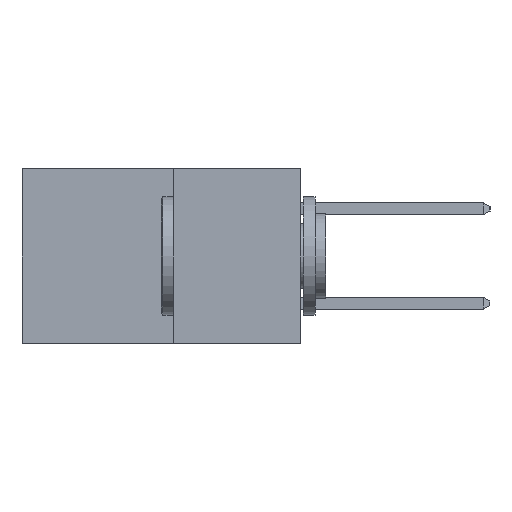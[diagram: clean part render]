
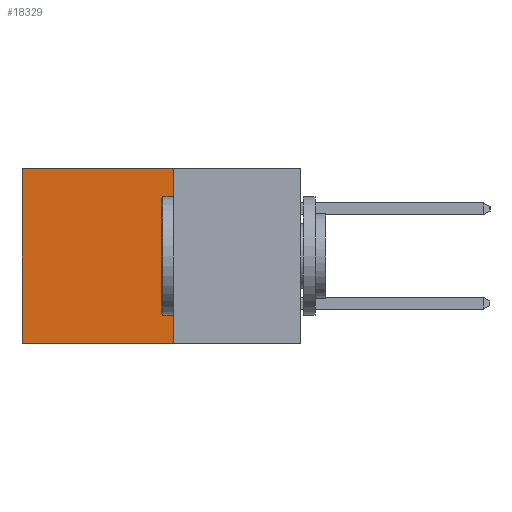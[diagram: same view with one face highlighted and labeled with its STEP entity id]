
A CAD part, left-side view. The second image highlights one B-rep face of the part: STEP entity #18329.
In plain terms, the highlighted planar face has unit normal (-1, 0, 0).
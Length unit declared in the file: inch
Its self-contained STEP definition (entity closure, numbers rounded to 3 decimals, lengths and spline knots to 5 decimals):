
#152 = EDGE_CURVE ( 'NONE', #6228, #7669, #28660, .T. ) ;
#1221 = CARTESIAN_POINT ( 'NONE',  ( 0.277, 0.27, -0.37 ) ) ;
#1982 = PLANE ( 'NONE',  #23885 ) ;
#2943 = DIRECTION ( 'NONE',  ( 0., 1., 0. ) ) ;
#3325 = DIRECTION ( 'NONE',  ( 0., 0., -1. ) ) ;
#4357 = DIRECTION ( 'NONE',  ( 0., 0., -1. ) ) ;
#4383 = ORIENTED_EDGE ( 'NONE', *, *, #19070, .F. ) ;
#5426 = CARTESIAN_POINT ( 'NONE',  ( 0.277, 0.59, -0.37 ) ) ;
#6228 = VERTEX_POINT ( 'NONE', #18841 ) ;
#7325 = FACE_OUTER_BOUND ( 'NONE', #9480, .T. ) ;
#7669 = VERTEX_POINT ( 'NONE', #28360 ) ;
#9480 = EDGE_LOOP ( 'NONE', ( #26126, #4383, #11478, #27191 ) ) ;
#9763 = EDGE_CURVE ( 'NONE', #6228, #13042, #27057, .T. ) ;
#10305 = VERTEX_POINT ( 'NONE', #5426 ) ;
#11478 = ORIENTED_EDGE ( 'NONE', *, *, #9763, .F. ) ;
#13042 = VERTEX_POINT ( 'NONE', #14444 ) ;
#14444 = CARTESIAN_POINT ( 'NONE',  ( 0.277, 0.27, -0.37 ) ) ;
#14736 = CARTESIAN_POINT ( 'NONE',  ( 0.277, 0.27, 0. ) ) ;
#15984 = EDGE_CURVE ( 'NONE', #7669, #10305, #28561, .T. ) ;
#17325 = CARTESIAN_POINT ( 'NONE',  ( 0.277, 0.27, -0.37 ) ) ;
#17965 = DIRECTION ( 'NONE',  ( 0., 1., 0. ) ) ;
#17975 = DIRECTION ( 'NONE',  ( 0., 0., -1. ) ) ;
#18202 = VECTOR ( 'NONE', #2943, 39.37008 ) ;
#18329 = ADVANCED_FACE ( 'NONE', ( #7325 ), #1982, .F. ) ;
#18751 = DIRECTION ( 'NONE',  ( 1., 0., 0. ) ) ;
#18841 = CARTESIAN_POINT ( 'NONE',  ( 0.277, 0.27, 0. ) ) ;
#19070 = EDGE_CURVE ( 'NONE', #13042, #10305, #23687, .T. ) ;
#22325 = CARTESIAN_POINT ( 'NONE',  ( 0.277, 0.59, -0.37 ) ) ;
#23687 = LINE ( 'NONE', #17325, #18202 ) ;
#23885 = AXIS2_PLACEMENT_3D ( 'NONE', #25713, #18751, #4357 ) ;
#25713 = CARTESIAN_POINT ( 'NONE',  ( 0.277, 0.27, -0.37 ) ) ;
#26126 = ORIENTED_EDGE ( 'NONE', *, *, #15984, .T. ) ;
#26312 = VECTOR ( 'NONE', #17975, 39.37008 ) ;
#26375 = VECTOR ( 'NONE', #3325, 39.37008 ) ;
#27057 = LINE ( 'NONE', #1221, #26312 ) ;
#27191 = ORIENTED_EDGE ( 'NONE', *, *, #152, .T. ) ;
#27199 = VECTOR ( 'NONE', #17965, 39.37008 ) ;
#28360 = CARTESIAN_POINT ( 'NONE',  ( 0.277, 0.59, 0. ) ) ;
#28561 = LINE ( 'NONE', #22325, #26375 ) ;
#28660 = LINE ( 'NONE', #14736, #27199 ) ;
